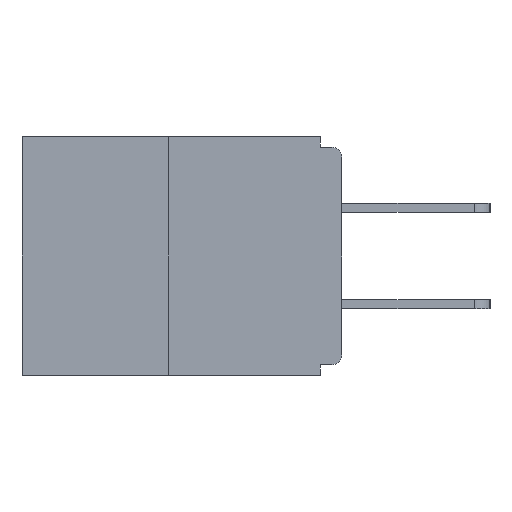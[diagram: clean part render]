
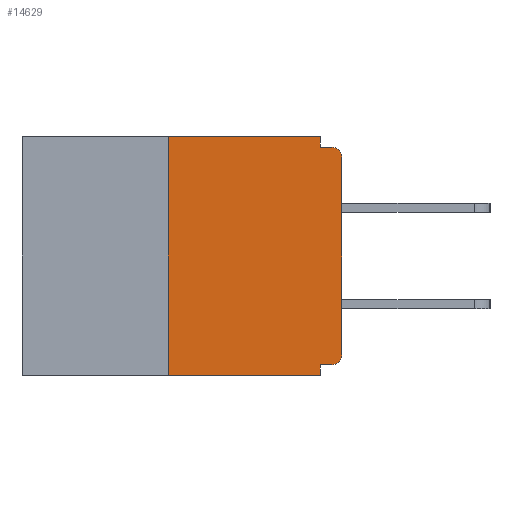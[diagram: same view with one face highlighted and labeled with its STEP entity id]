
A CAD part, left-side view. The second image highlights one B-rep face of the part: STEP entity #14629.
In plain terms, the highlighted planar face has unit normal (-1, 0, 0).
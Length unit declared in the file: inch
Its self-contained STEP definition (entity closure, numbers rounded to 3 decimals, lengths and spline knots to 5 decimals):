
#187 = VECTOR ( 'NONE', #6874, 39.37008 ) ;
#220 = DIRECTION ( 'NONE',  ( 1., 0., 0. ) ) ;
#230 = CARTESIAN_POINT ( 'NONE',  ( 0., 0.031, 0. ) ) ;
#305 = CARTESIAN_POINT ( 'NONE',  ( 0., 0.46, -0.343 ) ) ;
#1023 = VERTEX_POINT ( 'NONE', #11149 ) ;
#1036 = ORIENTED_EDGE ( 'NONE', *, *, #7789, .T. ) ;
#1574 = VERTEX_POINT ( 'NONE', #19060 ) ;
#1854 = VERTEX_POINT ( 'NONE', #14114 ) ;
#2414 = VECTOR ( 'NONE', #6945, 39.37008 ) ;
#2520 = DIRECTION ( 'NONE',  ( 0., 0., -1. ) ) ;
#2705 = ORIENTED_EDGE ( 'NONE', *, *, #18801, .F. ) ;
#2765 = DIRECTION ( 'NONE',  ( 0., 0., 1. ) ) ;
#2881 = CARTESIAN_POINT ( 'NONE',  ( 0., 0.015, -0.313 ) ) ;
#3018 = DIRECTION ( 'NONE',  ( 0., 0., -1. ) ) ;
#3054 = LINE ( 'NONE', #18731, #17730 ) ;
#3091 = CARTESIAN_POINT ( 'NONE',  ( 0., 0.031, -0.015 ) ) ;
#3123 = LINE ( 'NONE', #230, #17827 ) ;
#3289 = DIRECTION ( 'NONE',  ( 0., -1., 0. ) ) ;
#3348 = EDGE_LOOP ( 'NONE', ( #13807, #17476, #13464, #2705, #10080, #7937, #1036, #10059, #19126, #18703 ) ) ;
#4044 = VERTEX_POINT ( 'NONE', #17056 ) ;
#4748 = CARTESIAN_POINT ( 'NONE',  ( 0., 0.015, -0.015 ) ) ;
#5776 = CARTESIAN_POINT ( 'NONE',  ( 0., 0.015, -0.328 ) ) ;
#6076 = DIRECTION ( 'NONE',  ( 0., 1., 0. ) ) ;
#6093 = CARTESIAN_POINT ( 'NONE',  ( 0., 0., -0.313 ) ) ;
#6335 = DIRECTION ( 'NONE',  ( 0., 0., -1. ) ) ;
#6431 = PLANE ( 'NONE',  #10876 ) ;
#6559 = EDGE_CURVE ( 'NONE', #1854, #16075, #17049, .T. ) ;
#6863 = EDGE_CURVE ( 'NONE', #1854, #15348, #14932, .T. ) ;
#6874 = DIRECTION ( 'NONE',  ( 0., 0., -1. ) ) ;
#6945 = DIRECTION ( 'NONE',  ( 0., -1., 0. ) ) ;
#7252 = VERTEX_POINT ( 'NONE', #5776 ) ;
#7789 = EDGE_CURVE ( 'NONE', #16383, #1574, #3054, .T. ) ;
#7937 = ORIENTED_EDGE ( 'NONE', *, *, #14845, .T. ) ;
#9096 = CARTESIAN_POINT ( 'NONE',  ( 0., 0., -0.328 ) ) ;
#9098 = VECTOR ( 'NONE', #2765, 39.37008 ) ;
#10059 = ORIENTED_EDGE ( 'NONE', *, *, #14402, .T. ) ;
#10080 = ORIENTED_EDGE ( 'NONE', *, *, #10510, .F. ) ;
#10169 = DIRECTION ( 'NONE',  ( -1., 0., 0. ) ) ;
#10273 = CIRCLE ( 'NONE', #11530, 0.015 ) ;
#10510 = EDGE_CURVE ( 'NONE', #7252, #1023, #18213, .T. ) ;
#10801 = VECTOR ( 'NONE', #16949, 39.37008 ) ;
#10876 = AXIS2_PLACEMENT_3D ( 'NONE', #11154, #220, #6335 ) ;
#11149 = CARTESIAN_POINT ( 'NONE',  ( 0., 0.031, -0.328 ) ) ;
#11154 = CARTESIAN_POINT ( 'NONE',  ( 0., 0.46, 0. ) ) ;
#11207 = AXIS2_PLACEMENT_3D ( 'NONE', #12888, #10169, #2520 ) ;
#11283 = LINE ( 'NONE', #17400, #2414 ) ;
#11399 = VERTEX_POINT ( 'NONE', #3091 ) ;
#11530 = AXIS2_PLACEMENT_3D ( 'NONE', #2881, #14948, #16454 ) ;
#11592 = EDGE_CURVE ( 'NONE', #11399, #14193, #11283, .T. ) ;
#12436 = EDGE_CURVE ( 'NONE', #15348, #4044, #18458, .T. ) ;
#12619 = DIRECTION ( 'NONE',  ( 0., 0., 1. ) ) ;
#12888 = CARTESIAN_POINT ( 'NONE',  ( 0., 0.015, -0.03 ) ) ;
#13464 = ORIENTED_EDGE ( 'NONE', *, *, #6559, .T. ) ;
#13766 = CIRCLE ( 'NONE', #11207, 0.015 ) ;
#13807 = ORIENTED_EDGE ( 'NONE', *, *, #12436, .F. ) ;
#14114 = CARTESIAN_POINT ( 'NONE',  ( 0., 0.25, -0.343 ) ) ;
#14193 = VERTEX_POINT ( 'NONE', #4748 ) ;
#14340 = CARTESIAN_POINT ( 'NONE',  ( 0., 0.031, -0.343 ) ) ;
#14402 = EDGE_CURVE ( 'NONE', #1574, #14193, #13766, .T. ) ;
#14629 = ADVANCED_FACE ( 'NONE', ( #18787 ), #6431, .F. ) ;
#14845 = EDGE_CURVE ( 'NONE', #7252, #16383, #10273, .T. ) ;
#14932 = LINE ( 'NONE', #16537, #9098 ) ;
#14948 = DIRECTION ( 'NONE',  ( -1., 0., 0. ) ) ;
#15348 = VERTEX_POINT ( 'NONE', #18209 ) ;
#15804 = VECTOR ( 'NONE', #3289, 39.37008 ) ;
#16075 = VERTEX_POINT ( 'NONE', #14340 ) ;
#16212 = CARTESIAN_POINT ( 'NONE',  ( 0., 0.031, -0.343 ) ) ;
#16383 = VERTEX_POINT ( 'NONE', #6093 ) ;
#16454 = DIRECTION ( 'NONE',  ( 0., 0., -1. ) ) ;
#16515 = LINE ( 'NONE', #16212, #187 ) ;
#16537 = CARTESIAN_POINT ( 'NONE',  ( 0., 0.25, 0. ) ) ;
#16821 = VECTOR ( 'NONE', #6076, 39.37008 ) ;
#16949 = DIRECTION ( 'NONE',  ( 0., -1., 0. ) ) ;
#17049 = LINE ( 'NONE', #305, #15804 ) ;
#17056 = CARTESIAN_POINT ( 'NONE',  ( 0., 0.031, 0. ) ) ;
#17400 = CARTESIAN_POINT ( 'NONE',  ( 0., 0., -0.015 ) ) ;
#17476 = ORIENTED_EDGE ( 'NONE', *, *, #6863, .F. ) ;
#17730 = VECTOR ( 'NONE', #12619, 39.37008 ) ;
#17731 = EDGE_CURVE ( 'NONE', #4044, #11399, #3123, .T. ) ;
#17827 = VECTOR ( 'NONE', #3018, 39.37008 ) ;
#18209 = CARTESIAN_POINT ( 'NONE',  ( 0., 0.25, 0. ) ) ;
#18213 = LINE ( 'NONE', #9096, #16821 ) ;
#18357 = CARTESIAN_POINT ( 'NONE',  ( 0., 0.46, 0. ) ) ;
#18458 = LINE ( 'NONE', #18357, #10801 ) ;
#18703 = ORIENTED_EDGE ( 'NONE', *, *, #17731, .F. ) ;
#18731 = CARTESIAN_POINT ( 'NONE',  ( 0., 0., 0. ) ) ;
#18787 = FACE_OUTER_BOUND ( 'NONE', #3348, .T. ) ;
#18801 = EDGE_CURVE ( 'NONE', #1023, #16075, #16515, .T. ) ;
#19060 = CARTESIAN_POINT ( 'NONE',  ( 0., 0., -0.03 ) ) ;
#19126 = ORIENTED_EDGE ( 'NONE', *, *, #11592, .F. ) ;
